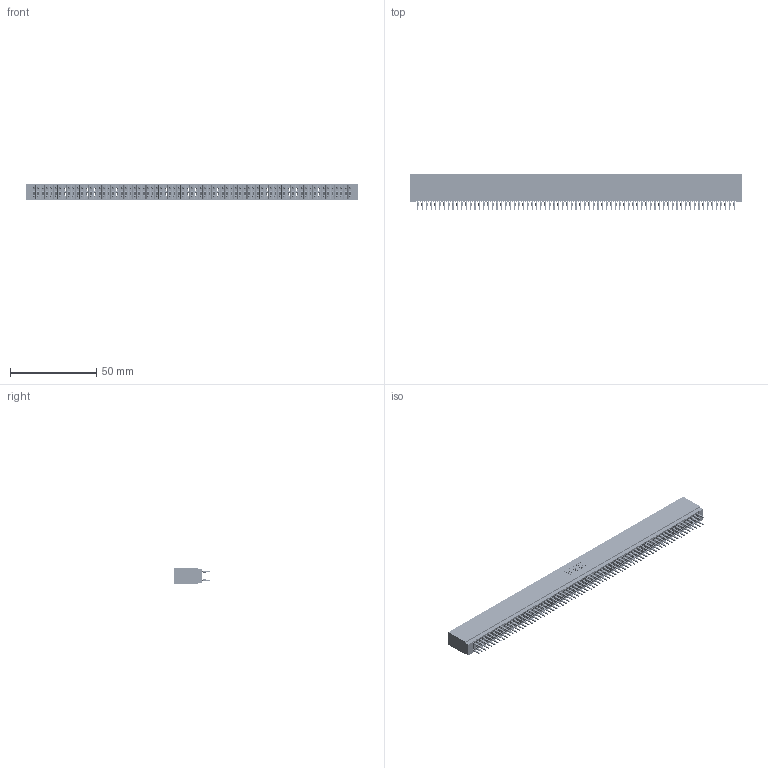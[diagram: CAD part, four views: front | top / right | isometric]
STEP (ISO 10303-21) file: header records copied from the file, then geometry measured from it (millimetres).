
FILE_DESCRIPTION (( 'STEP AP203' ), '1' );
FILE_NAME ('745-146-560-201.STEP', '2026-02-27T04:39:37', ( '' ), ( '' ), 'SwSTEP 2.0', 'SolidWorks 2023', '' );
FILE_SCHEMA (( 'CONFIG_CONTROL_DESIGN' ));
Length unit declared in the file: millimetre
Products named in the file (3): 745 Part_Insulator Option - 01; 745-292-001_560; 745-146-560-201
Assembly tree (147 placements, depth 2):
  745-146-560-201
    745 Part_Insulator Option - 01
    745-292-001_560  x146
Bounding box: 192.02 x 21.22 x 8.89 mm (x, y, z)
Volume: 17646.2 mm3; surface area: 38893.6 mm2
Topology: 147 solids, 147 shells, 14476 faces, 39605 edges, 25138 vertices
Faces by surface type: plane 7501, cylinder 3179, bspline 2920, torus 876
Entity records: 118988 total; most frequent: CARTESIAN_POINT 21133, ORIENTED_EDGE 20630, DIRECTION 17999, EDGE_CURVE 10315, LINE 9687, VECTOR 9687, VERTEX_POINT 6578, AXIS2_PLACEMENT_3D 4156
